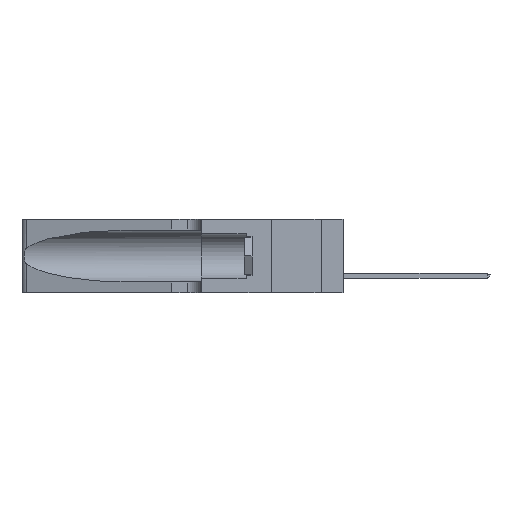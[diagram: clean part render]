
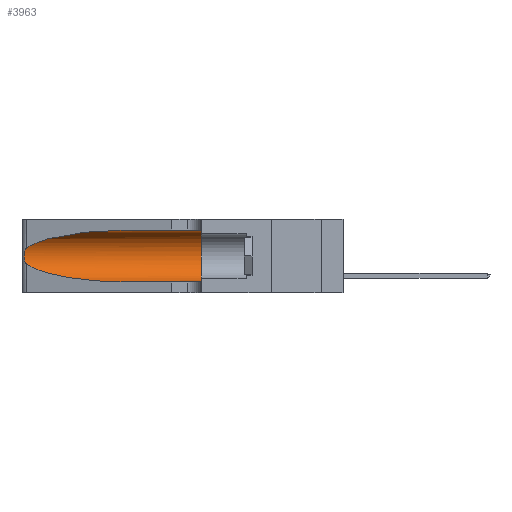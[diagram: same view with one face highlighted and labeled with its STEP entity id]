
A CAD part, left-side view. The second image highlights one B-rep face of the part: STEP entity #3963.
In plain terms, the highlighted cylindrical face has radius 3.308 mm (diameter 6.617 mm), a partial arc.
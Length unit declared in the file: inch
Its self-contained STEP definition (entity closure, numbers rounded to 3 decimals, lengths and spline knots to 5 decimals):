
#396 = EDGE_CURVE ( 'NONE', #38524, #24539, #14251, .T. ) ;
#1797 = CARTESIAN_POINT ( 'NONE',  ( 0.25487, 1.22718, 0.14631 ) ) ;
#2800 = CARTESIAN_POINT ( 'NONE',  ( 0.26075, 1.23896, 0.19203 ) ) ;
#2920 = CARTESIAN_POINT ( 'NONE',  ( 0.1305, 1.61858, 0.185 ) ) ;
#3237 = CARTESIAN_POINT ( 'NONE',  ( 0.25856, 1.23593, 0.16098 ) ) ;
#3963 = ADVANCED_FACE ( 'NONE', ( #13385 ), #41614, .F. ) ;
#4237 = ORIENTED_EDGE ( 'NONE', *, *, #36511, .T. ) ;
#4753 = AXIS2_PLACEMENT_3D ( 'NONE', #12754, #5941, #15994 ) ;
#4807 = EDGE_CURVE ( 'NONE', #24861, #30244, #32742, .T. ) ;
#4891 = VERTEX_POINT ( 'NONE', #17056 ) ;
#4984 = ORIENTED_EDGE ( 'NONE', *, *, #34148, .T. ) ;
#5194 = CARTESIAN_POINT ( 'NONE',  ( 0.1305, 1.61858, 0.31525 ) ) ;
#5941 = DIRECTION ( 'NONE',  ( 0., 1., 0. ) ) ;
#6520 = EDGE_CURVE ( 'NONE', #24539, #4891, #29349, .T. ) ;
#6740 = CARTESIAN_POINT ( 'NONE',  ( 0.1305, 1.61858, 0.05475 ) ) ;
#6982 = DIRECTION ( 'NONE',  ( 0., -1., 0. ) ) ;
#7854 = ORIENTED_EDGE ( 'NONE', *, *, #4807, .F. ) ;
#8304 = CARTESIAN_POINT ( 'NONE',  ( 0.25487, 1.22718, 0.22369 ) ) ;
#8596 = VERTEX_POINT ( 'NONE', #27850 ) ;
#8688 = LINE ( 'NONE', #5194, #43154 ) ;
#9538 = CARTESIAN_POINT ( 'NONE',  ( 0.25487, 1.22718, 0.22369 ) ) ;
#9672 = CARTESIAN_POINT ( 'NONE',  ( 0.26018, 1.23835, 0.19895 ) ) ;
#9881 = ORIENTED_EDGE ( 'NONE', *, *, #6520, .T. ) ;
#10867 = AXIS2_PLACEMENT_3D ( 'NONE', #2920, #39929, #19988 ) ;
#12754 = CARTESIAN_POINT ( 'NONE',  ( 0.1305, 0.35, 0.185 ) ) ;
#13385 = FACE_OUTER_BOUND ( 'NONE', #15106, .T. ) ;
#13511 = ORIENTED_EDGE ( 'NONE', *, *, #396, .T. ) ;
#14251 = B_SPLINE_CURVE_WITH_KNOTS ( 'NONE', 3,
 ( #9538, #23141, #19739, #22853, #16220, #9672, #2800, #39379, #42791, #3237, #22998, #26073, #42626, #39689 ),
 .UNSPECIFIED., .F., .F.,
 ( 4, 2, 2, 2, 2, 2, 4 ),
 ( 0., 0.00027, 0.00053, 0.00107, 0.0016, 0.00187, 0.00214 ),
 .UNSPECIFIED. ) ;
#15106 = EDGE_LOOP ( 'NONE', ( #4984, #13511, #9881, #4237, #7854, #20733 ) ) ;
#15994 = DIRECTION ( 'NONE',  ( 0., 0., 1. ) ) ;
#16220 = CARTESIAN_POINT ( 'NONE',  ( 0.25854, 1.2359, 0.20912 ) ) ;
#17056 = CARTESIAN_POINT ( 'NONE',  ( 0.1305, 0.72297, 0.05475 ) ) ;
#19317 = CARTESIAN_POINT ( 'NONE',  ( 0.1305, 0.72297, 0.31525 ) ) ;
#19739 = CARTESIAN_POINT ( 'NONE',  ( 0.25639, 1.23184, 0.21858 ) ) ;
#19988 = DIRECTION ( 'NONE',  ( 0., 0., -1. ) ) ;
#20292 = CARTESIAN_POINT ( 'NONE',  ( 0.2373, 1.15595, 0.08982 ) ) ;
#20733 = ORIENTED_EDGE ( 'NONE', *, *, #36253, .F. ) ;
#22853 = CARTESIAN_POINT ( 'NONE',  ( 0.25787, 1.23484, 0.2124 ) ) ;
#22998 = CARTESIAN_POINT ( 'NONE',  ( 0.25789, 1.23486, 0.15765 ) ) ;
#23141 = CARTESIAN_POINT ( 'NONE',  ( 0.25555, 1.22994, 0.2215 ) ) ;
#24539 = VERTEX_POINT ( 'NONE', #1797 ) ;
#24688 = CARTESIAN_POINT ( 'NONE',  ( 0.25487, 1.22718, 0.14631 ) ) ;
#24861 = VERTEX_POINT ( 'NONE', #40787 ) ;
#26073 = CARTESIAN_POINT ( 'NONE',  ( 0.25639, 1.23186, 0.15144 ) ) ;
#26856 = CARTESIAN_POINT ( 'NONE',  ( 0.1305, 0.72297, 0.05475 ) ) ;
#27850 = CARTESIAN_POINT ( 'NONE',  ( 0.1305, 0.72297, 0.31525 ) ) ;
#27918 = CARTESIAN_POINT ( 'NONE',  ( 0.1305, 0.35, 0.05475 ) ) ;
#27975 = VECTOR ( 'NONE', #6982, 39.37008 ) ;
#29349 =( BOUNDED_CURVE ( )  B_SPLINE_CURVE ( 3, ( #24688, #20292, #38924, #26856 ),
 .UNSPECIFIED., .F., .T. ) 
 B_SPLINE_CURVE_WITH_KNOTS ( ( 4, 4 ),
 ( 3.44316, 4.71239 ),
 .UNSPECIFIED. ) 
 CURVE ( )  GEOMETRIC_REPRESENTATION_ITEM ( )  RATIONAL_B_SPLINE_CURVE ( ( 1., 0.87, 0.87, 1. ) ) 
 REPRESENTATION_ITEM ( '' )  );
#29555 = LINE ( 'NONE', #6740, #27975 ) ;
#30244 = VERTEX_POINT ( 'NONE', #27918 ) ;
#32742 = CIRCLE ( 'NONE', #4753, 0.13025 ) ;
#33059 = DIRECTION ( 'NONE',  ( 0., -1., 0. ) ) ;
#34148 = EDGE_CURVE ( 'NONE', #8596, #38524, #34375, .T. ) ;
#34375 =( BOUNDED_CURVE ( )  B_SPLINE_CURVE ( 3, ( #19317, #39109, #43080, #42485 ),
 .UNSPECIFIED., .F., .T. ) 
 B_SPLINE_CURVE_WITH_KNOTS ( ( 4, 4 ),
 ( 1.5708, 2.84003 ),
 .UNSPECIFIED. ) 
 CURVE ( )  GEOMETRIC_REPRESENTATION_ITEM ( )  RATIONAL_B_SPLINE_CURVE ( ( 1., 0.87, 0.87, 1. ) ) 
 REPRESENTATION_ITEM ( '' )  );
#36253 = EDGE_CURVE ( 'NONE', #8596, #24861, #8688, .T. ) ;
#36511 = EDGE_CURVE ( 'NONE', #4891, #30244, #29555, .T. ) ;
#38524 = VERTEX_POINT ( 'NONE', #8304 ) ;
#38924 = CARTESIAN_POINT ( 'NONE',  ( 0.18966, 0.96281, 0.05475 ) ) ;
#39109 = CARTESIAN_POINT ( 'NONE',  ( 0.18966, 0.96281, 0.31525 ) ) ;
#39379 = CARTESIAN_POINT ( 'NONE',  ( 0.26075, 1.23896, 0.178 ) ) ;
#39689 = CARTESIAN_POINT ( 'NONE',  ( 0.25487, 1.22718, 0.14631 ) ) ;
#39929 = DIRECTION ( 'NONE',  ( 0., -1., 0. ) ) ;
#40787 = CARTESIAN_POINT ( 'NONE',  ( 0.1305, 0.35, 0.31525 ) ) ;
#41614 = CYLINDRICAL_SURFACE ( 'NONE', #10867, 0.13025 ) ;
#42485 = CARTESIAN_POINT ( 'NONE',  ( 0.25487, 1.22718, 0.22369 ) ) ;
#42626 = CARTESIAN_POINT ( 'NONE',  ( 0.25555, 1.22993, 0.14849 ) ) ;
#42791 = CARTESIAN_POINT ( 'NONE',  ( 0.26017, 1.23833, 0.17102 ) ) ;
#43080 = CARTESIAN_POINT ( 'NONE',  ( 0.2373, 1.15595, 0.28018 ) ) ;
#43154 = VECTOR ( 'NONE', #33059, 39.37008 ) ;
